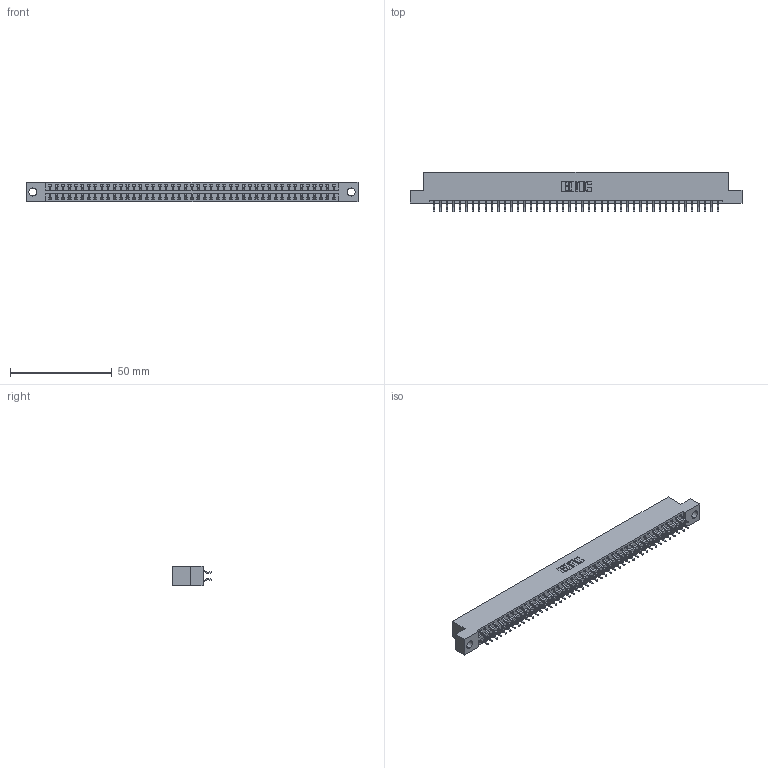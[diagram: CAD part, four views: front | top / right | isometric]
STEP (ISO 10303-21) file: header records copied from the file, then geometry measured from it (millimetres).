
FILE_DESCRIPTION (( 'STEP AP203' ), '1' );
FILE_NAME ('396-090-556-204.STEP', '2019-10-31T02:12:06', ( '' ), ( '' ), 'SwSTEP 2.0', 'SolidWorks 2016', '' );
FILE_SCHEMA (( 'CONFIG_CONTROL_DESIGN' ));
Length unit declared in the file: inch
Products named in the file (3): 346 Part_Flush Mounting Lugs - 0.156 Dia-TH; 345-292-001_556 Tail; 396-090-556-204
Assembly tree (91 placements, depth 2):
  396-090-556-204
    346 Part_Flush Mounting Lugs - 0.156 Dia-TH
    345-292-001_556 Tail  x90
Bounding box: 163.45 x 19.57 x 9.4 mm (x, y, z)
Volume: 15870.2 mm3; surface area: 21591.5 mm2
Topology: 91 solids, 91 shells, 5342 faces, 15899 edges, 10478 vertices
Faces by surface type: plane 3586, cylinder 1756
Entity records: 29187 total; most frequent: CARTESIAN_POINT 4820, ORIENTED_EDGE 4742, DIRECTION 4287, EDGE_CURVE 2371, LINE 2051, VECTOR 2051, VERTEX_POINT 1578, AXIS2_PLACEMENT_3D 1118
